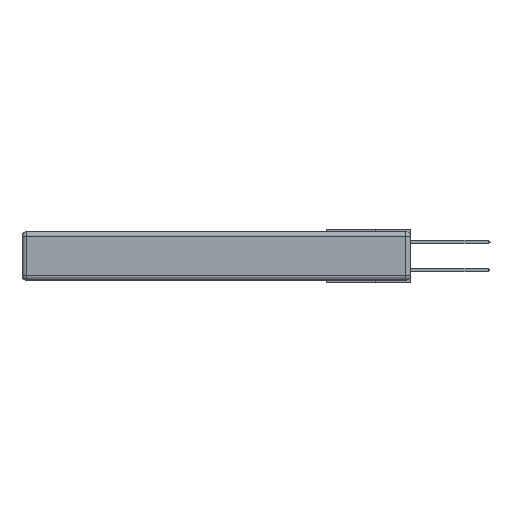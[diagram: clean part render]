
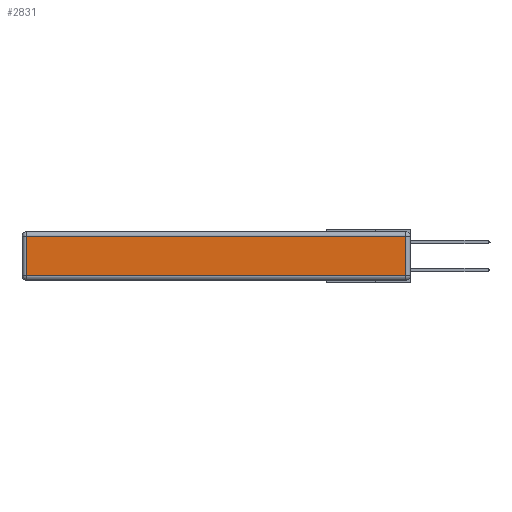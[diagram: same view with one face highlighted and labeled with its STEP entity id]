
A CAD part, left-side view. The second image highlights one B-rep face of the part: STEP entity #2831.
In plain terms, the highlighted planar face has unit normal (-1, 0, 0).
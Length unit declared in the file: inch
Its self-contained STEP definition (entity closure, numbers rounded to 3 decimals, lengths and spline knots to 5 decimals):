
#227 = PLANE ( 'NONE',  #7510 ) ;
#519 = VERTEX_POINT ( 'NONE', #4986 ) ;
#1177 = FACE_OUTER_BOUND ( 'NONE', #10732, .T. ) ;
#1342 = VECTOR ( 'NONE', #3812, 39.37008 ) ;
#1540 = CARTESIAN_POINT ( 'NONE',  ( 0., 0.03, -0.03 ) ) ;
#2428 = ORIENTED_EDGE ( 'NONE', *, *, #12806, .T. ) ;
#2429 = VERTEX_POINT ( 'NONE', #12496 ) ;
#2544 = LINE ( 'NONE', #8225, #4572 ) ;
#2831 = ADVANCED_FACE ( 'NONE', ( #1177 ), #227, .T. ) ;
#2998 = CARTESIAN_POINT ( 'NONE',  ( 0., 0., -0.343 ) ) ;
#3812 = DIRECTION ( 'NONE',  ( 0., 1., 0. ) ) ;
#4572 = VECTOR ( 'NONE', #9461, 39.37008 ) ;
#4614 = CARTESIAN_POINT ( 'NONE',  ( 0., 0.03, -0.313 ) ) ;
#4986 = CARTESIAN_POINT ( 'NONE',  ( 0., 2.72, -0.03 ) ) ;
#5275 = CARTESIAN_POINT ( 'NONE',  ( 0., 0., -0.313 ) ) ;
#5479 = VECTOR ( 'NONE', #12447, 39.37008 ) ;
#5545 = DIRECTION ( 'NONE',  ( 0., 0., 1. ) ) ;
#5710 = ORIENTED_EDGE ( 'NONE', *, *, #10896, .T. ) ;
#6279 = ORIENTED_EDGE ( 'NONE', *, *, #12521, .T. ) ;
#6545 = LINE ( 'NONE', #13197, #1342 ) ;
#6715 = VERTEX_POINT ( 'NONE', #4614 ) ;
#7510 = AXIS2_PLACEMENT_3D ( 'NONE', #2998, #7794, #10142 ) ;
#7794 = DIRECTION ( 'NONE',  ( -1., 0., 0. ) ) ;
#8225 = CARTESIAN_POINT ( 'NONE',  ( 0., 2.72, -0.343 ) ) ;
#9461 = DIRECTION ( 'NONE',  ( 0., 0., -1. ) ) ;
#9872 = VECTOR ( 'NONE', #5545, 39.37008 ) ;
#10142 = DIRECTION ( 'NONE',  ( 0., 0., 1. ) ) ;
#10732 = EDGE_LOOP ( 'NONE', ( #11728, #2428, #6279, #5710 ) ) ;
#10896 = EDGE_CURVE ( 'NONE', #519, #2429, #2544, .T. ) ;
#11356 = LINE ( 'NONE', #13819, #9872 ) ;
#11728 = ORIENTED_EDGE ( 'NONE', *, *, #14007, .T. ) ;
#12063 = VERTEX_POINT ( 'NONE', #1540 ) ;
#12447 = DIRECTION ( 'NONE',  ( 0., -1., 0. ) ) ;
#12496 = CARTESIAN_POINT ( 'NONE',  ( 0., 2.72, -0.313 ) ) ;
#12521 = EDGE_CURVE ( 'NONE', #12063, #519, #6545, .T. ) ;
#12700 = LINE ( 'NONE', #5275, #5479 ) ;
#12806 = EDGE_CURVE ( 'NONE', #6715, #12063, #11356, .T. ) ;
#13197 = CARTESIAN_POINT ( 'NONE',  ( 0., 2.75, -0.03 ) ) ;
#13819 = CARTESIAN_POINT ( 'NONE',  ( 0., 0.03, -0.343 ) ) ;
#14007 = EDGE_CURVE ( 'NONE', #2429, #6715, #12700, .T. ) ;
